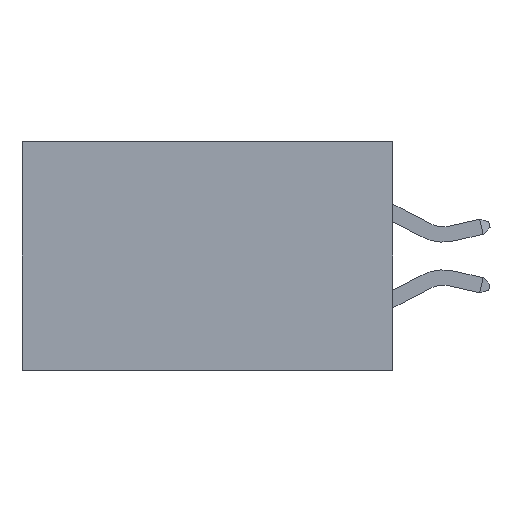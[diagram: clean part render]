
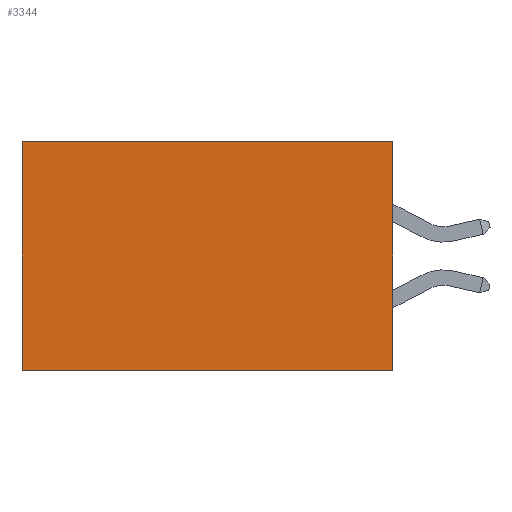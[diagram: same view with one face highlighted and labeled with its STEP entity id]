
A CAD part, left-side view. The second image highlights one B-rep face of the part: STEP entity #3344.
In plain terms, the highlighted planar face has unit normal (-1, 0, 0).
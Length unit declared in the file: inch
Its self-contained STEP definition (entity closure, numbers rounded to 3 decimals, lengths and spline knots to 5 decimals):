
#1466 = CARTESIAN_POINT ( 'NONE',  ( 0.2875, 0.6, 0. ) ) ;
#1473 = EDGE_CURVE ( 'NONE', #20284, #11400, #3546, .T. ) ;
#1636 = VERTEX_POINT ( 'NONE', #1466 ) ;
#2676 = CARTESIAN_POINT ( 'NONE',  ( 0.2875, 0., 0. ) ) ;
#3020 = EDGE_CURVE ( 'NONE', #11400, #8145, #13271, .T. ) ;
#3311 = CARTESIAN_POINT ( 'NONE',  ( 0.2875, 0., -0.37 ) ) ;
#3344 = ADVANCED_FACE ( 'NONE', ( #18621 ), #4138, .F. ) ;
#3546 = LINE ( 'NONE', #2676, #10768 ) ;
#4138 = PLANE ( 'NONE',  #9763 ) ;
#4268 = LINE ( 'NONE', #13475, #12491 ) ;
#4405 = CARTESIAN_POINT ( 'NONE',  ( 0.2875, 0., 0. ) ) ;
#6474 = LINE ( 'NONE', #16855, #14116 ) ;
#8145 = VERTEX_POINT ( 'NONE', #13091 ) ;
#8631 = EDGE_LOOP ( 'NONE', ( #15759, #15282, #11871, #18565 ) ) ;
#9703 = EDGE_CURVE ( 'NONE', #1636, #8145, #6474, .T. ) ;
#9763 = AXIS2_PLACEMENT_3D ( 'NONE', #20071, #21038, #21163 ) ;
#10768 = VECTOR ( 'NONE', #20736, 39.37008 ) ;
#11400 = VERTEX_POINT ( 'NONE', #3311 ) ;
#11871 = ORIENTED_EDGE ( 'NONE', *, *, #1473, .F. ) ;
#12491 = VECTOR ( 'NONE', #15113, 39.37008 ) ;
#12633 = EDGE_CURVE ( 'NONE', #20284, #1636, #4268, .T. ) ;
#13091 = CARTESIAN_POINT ( 'NONE',  ( 0.2875, 0.6, -0.37 ) ) ;
#13271 = LINE ( 'NONE', #16478, #20374 ) ;
#13475 = CARTESIAN_POINT ( 'NONE',  ( 0.2875, 0., 0. ) ) ;
#14116 = VECTOR ( 'NONE', #18492, 39.37008 ) ;
#15113 = DIRECTION ( 'NONE',  ( 0., 1., 0. ) ) ;
#15282 = ORIENTED_EDGE ( 'NONE', *, *, #3020, .F. ) ;
#15759 = ORIENTED_EDGE ( 'NONE', *, *, #9703, .T. ) ;
#16478 = CARTESIAN_POINT ( 'NONE',  ( 0.2875, 0., -0.37 ) ) ;
#16632 = DIRECTION ( 'NONE',  ( 0., 1., 0. ) ) ;
#16855 = CARTESIAN_POINT ( 'NONE',  ( 0.2875, 0.6, 0. ) ) ;
#18492 = DIRECTION ( 'NONE',  ( 0., 0., -1. ) ) ;
#18565 = ORIENTED_EDGE ( 'NONE', *, *, #12633, .T. ) ;
#18621 = FACE_OUTER_BOUND ( 'NONE', #8631, .T. ) ;
#20071 = CARTESIAN_POINT ( 'NONE',  ( 0.2875, 0., 0. ) ) ;
#20284 = VERTEX_POINT ( 'NONE', #4405 ) ;
#20374 = VECTOR ( 'NONE', #16632, 39.37008 ) ;
#20736 = DIRECTION ( 'NONE',  ( 0., 0., -1. ) ) ;
#21038 = DIRECTION ( 'NONE',  ( 1., 0., 0. ) ) ;
#21163 = DIRECTION ( 'NONE',  ( 0., 0., -1. ) ) ;
